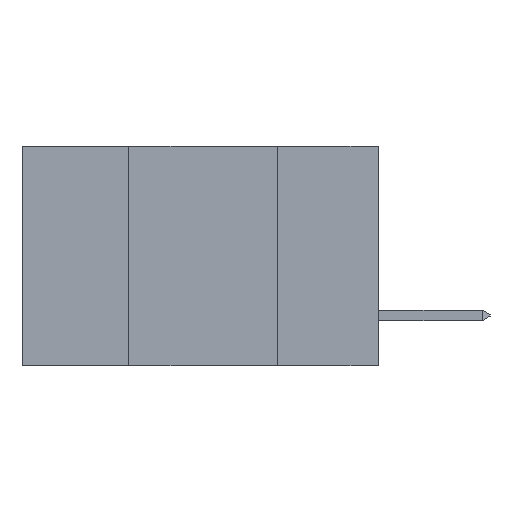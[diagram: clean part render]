
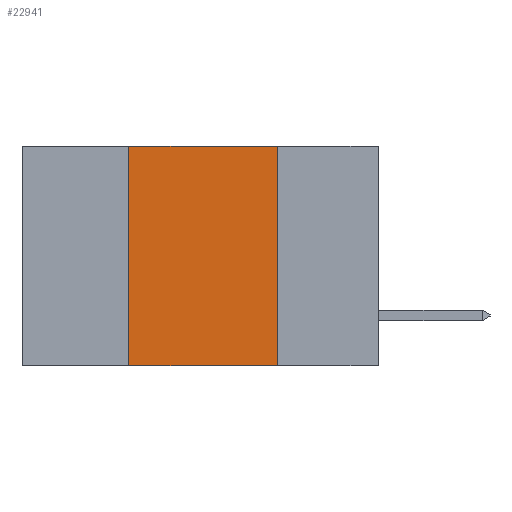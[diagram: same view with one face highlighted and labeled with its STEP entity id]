
A CAD part, left-side view. The second image highlights one B-rep face of the part: STEP entity #22941.
In plain terms, the highlighted planar face has unit normal (-1, 0, 0).
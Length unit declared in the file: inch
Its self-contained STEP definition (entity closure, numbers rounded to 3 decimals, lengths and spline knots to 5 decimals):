
#981 = CARTESIAN_POINT ( 'NONE',  ( 0., 0.42, -0.37 ) ) ;
#1235 = CARTESIAN_POINT ( 'NONE',  ( 0., 0.42, 0. ) ) ;
#1359 = DIRECTION ( 'NONE',  ( 0., 0., 1. ) ) ;
#1599 = DIRECTION ( 'NONE',  ( 0., -1., 0. ) ) ;
#1777 = CARTESIAN_POINT ( 'NONE',  ( 0., 0.6, 0. ) ) ;
#2398 = FACE_OUTER_BOUND ( 'NONE', #17186, .T. ) ;
#2652 = EDGE_CURVE ( 'NONE', #14764, #26071, #17775, .T. ) ;
#2731 = CARTESIAN_POINT ( 'NONE',  ( 0., 0.6, -0.37 ) ) ;
#3807 = PLANE ( 'NONE',  #22673 ) ;
#3818 = ORIENTED_EDGE ( 'NONE', *, *, #25108, .F. ) ;
#5023 = DIRECTION ( 'NONE',  ( 0., -1., 0. ) ) ;
#5871 = LINE ( 'NONE', #15703, #17142 ) ;
#6083 = CARTESIAN_POINT ( 'NONE',  ( 0., 0.6, 0. ) ) ;
#6659 = ORIENTED_EDGE ( 'NONE', *, *, #25273, .T. ) ;
#6696 = DIRECTION ( 'NONE',  ( 0., 0., -1. ) ) ;
#6716 = EDGE_CURVE ( 'NONE', #12132, #14764, #16181, .T. ) ;
#6899 = LINE ( 'NONE', #2731, #12938 ) ;
#8067 = ORIENTED_EDGE ( 'NONE', *, *, #2652, .F. ) ;
#9060 = VERTEX_POINT ( 'NONE', #22958 ) ;
#10176 = VECTOR ( 'NONE', #1359, 39.37008 ) ;
#10629 = DIRECTION ( 'NONE',  ( 0., 0., -1. ) ) ;
#12132 = VERTEX_POINT ( 'NONE', #981 ) ;
#12694 = CARTESIAN_POINT ( 'NONE',  ( 0., 0.42, 0. ) ) ;
#12938 = VECTOR ( 'NONE', #5023, 39.37008 ) ;
#14764 = VERTEX_POINT ( 'NONE', #1235 ) ;
#15703 = CARTESIAN_POINT ( 'NONE',  ( 0., 0.17, 0. ) ) ;
#16181 = LINE ( 'NONE', #12694, #10176 ) ;
#17142 = VECTOR ( 'NONE', #6696, 39.37008 ) ;
#17186 = EDGE_LOOP ( 'NONE', ( #3818, #8067, #26518, #6659 ) ) ;
#17775 = LINE ( 'NONE', #1777, #28735 ) ;
#21292 = CARTESIAN_POINT ( 'NONE',  ( 0., 0.17, 0. ) ) ;
#22673 = AXIS2_PLACEMENT_3D ( 'NONE', #6083, #24021, #10629 ) ;
#22941 = ADVANCED_FACE ( 'NONE', ( #2398 ), #3807, .F. ) ;
#22958 = CARTESIAN_POINT ( 'NONE',  ( 0., 0.17, -0.37 ) ) ;
#24021 = DIRECTION ( 'NONE',  ( 1., 0., 0. ) ) ;
#25108 = EDGE_CURVE ( 'NONE', #26071, #9060, #5871, .T. ) ;
#25273 = EDGE_CURVE ( 'NONE', #12132, #9060, #6899, .T. ) ;
#26071 = VERTEX_POINT ( 'NONE', #21292 ) ;
#26518 = ORIENTED_EDGE ( 'NONE', *, *, #6716, .F. ) ;
#28735 = VECTOR ( 'NONE', #1599, 39.37008 ) ;
